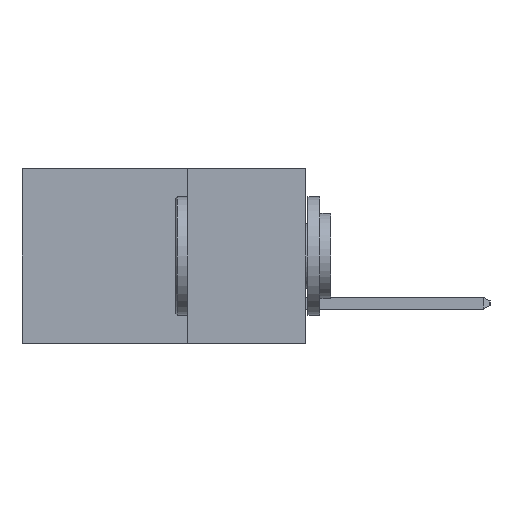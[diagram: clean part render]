
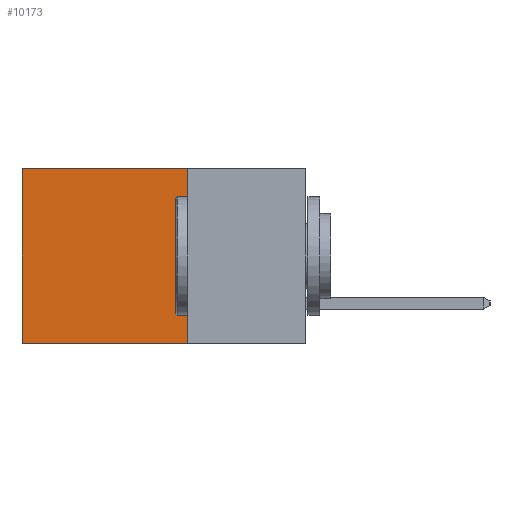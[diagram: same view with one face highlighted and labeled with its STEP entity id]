
A CAD part, left-side view. The second image highlights one B-rep face of the part: STEP entity #10173.
In plain terms, the highlighted planar face has unit normal (-1, 0, 0).
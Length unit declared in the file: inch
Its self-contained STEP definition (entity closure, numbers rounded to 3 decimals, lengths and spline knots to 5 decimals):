
#823 = VERTEX_POINT ( 'NONE', #3474 ) ;
#1108 = DIRECTION ( 'NONE',  ( 0., 0., -1. ) ) ;
#1689 = VERTEX_POINT ( 'NONE', #9235 ) ;
#2016 = EDGE_CURVE ( 'NONE', #7792, #10537, #12760, .T. ) ;
#3118 = AXIS2_PLACEMENT_3D ( 'NONE', #13461, #7530, #1108 ) ;
#3203 = EDGE_CURVE ( 'NONE', #1689, #823, #11346, .T. ) ;
#3322 = CARTESIAN_POINT ( 'NONE',  ( 0.298, 0.25, 0. ) ) ;
#3356 = EDGE_CURVE ( 'NONE', #10537, #823, #9487, .T. ) ;
#3474 = CARTESIAN_POINT ( 'NONE',  ( 0.298, 0.6, -0.37 ) ) ;
#4284 = PLANE ( 'NONE',  #3118 ) ;
#4596 = VECTOR ( 'NONE', #7913, 39.37008 ) ;
#4774 = CARTESIAN_POINT ( 'NONE',  ( 0.298, 0.25, 0. ) ) ;
#5224 = EDGE_LOOP ( 'NONE', ( #9109, #8334, #7827, #5965 ) ) ;
#5965 = ORIENTED_EDGE ( 'NONE', *, *, #6677, .T. ) ;
#6250 = VECTOR ( 'NONE', #8268, 39.37008 ) ;
#6675 = CARTESIAN_POINT ( 'NONE',  ( 0.298, 0.25, 0. ) ) ;
#6677 = EDGE_CURVE ( 'NONE', #7792, #1689, #10350, .T. ) ;
#6728 = VECTOR ( 'NONE', #13395, 39.37008 ) ;
#7088 = CARTESIAN_POINT ( 'NONE',  ( 0.298, 0.25, -0.37 ) ) ;
#7530 = DIRECTION ( 'NONE',  ( 1., 0., 0. ) ) ;
#7792 = VERTEX_POINT ( 'NONE', #3322 ) ;
#7827 = ORIENTED_EDGE ( 'NONE', *, *, #2016, .F. ) ;
#7913 = DIRECTION ( 'NONE',  ( 0., 0., -1. ) ) ;
#8268 = DIRECTION ( 'NONE',  ( 0., 0., -1. ) ) ;
#8334 = ORIENTED_EDGE ( 'NONE', *, *, #3356, .F. ) ;
#9109 = ORIENTED_EDGE ( 'NONE', *, *, #3203, .T. ) ;
#9235 = CARTESIAN_POINT ( 'NONE',  ( 0.298, 0.6, 0. ) ) ;
#9487 = LINE ( 'NONE', #13327, #6728 ) ;
#10173 = ADVANCED_FACE ( 'NONE', ( #12948 ), #4284, .F. ) ;
#10350 = LINE ( 'NONE', #4774, #12340 ) ;
#10537 = VERTEX_POINT ( 'NONE', #7088 ) ;
#11346 = LINE ( 'NONE', #11402, #6250 ) ;
#11402 = CARTESIAN_POINT ( 'NONE',  ( 0.298, 0.6, 0. ) ) ;
#11948 = DIRECTION ( 'NONE',  ( 0., 1., 0. ) ) ;
#12340 = VECTOR ( 'NONE', #11948, 39.37008 ) ;
#12760 = LINE ( 'NONE', #6675, #4596 ) ;
#12948 = FACE_OUTER_BOUND ( 'NONE', #5224, .T. ) ;
#13327 = CARTESIAN_POINT ( 'NONE',  ( 0.298, 0.25, -0.37 ) ) ;
#13395 = DIRECTION ( 'NONE',  ( 0., 1., 0. ) ) ;
#13461 = CARTESIAN_POINT ( 'NONE',  ( 0.298, 0.25, 0. ) ) ;
